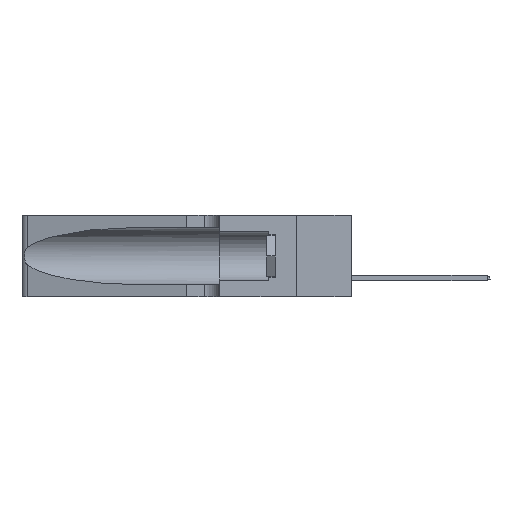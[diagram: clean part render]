
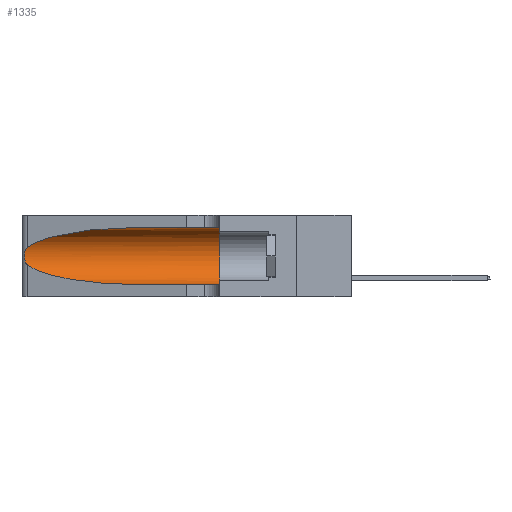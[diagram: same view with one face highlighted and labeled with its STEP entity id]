
A CAD part, left-side view. The second image highlights one B-rep face of the part: STEP entity #1335.
In plain terms, the highlighted cylindrical face has radius 3.308 mm (diameter 6.617 mm), a partial arc.
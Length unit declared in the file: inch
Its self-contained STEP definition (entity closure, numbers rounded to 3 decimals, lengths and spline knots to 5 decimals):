
#7 = CARTESIAN_POINT ( 'NONE',  ( 0.25487, 1.22718, 0.22369 ) ) ;
#128 = LINE ( 'NONE', #35612, #27657 ) ;
#715 = CARTESIAN_POINT ( 'NONE',  ( 0.25487, 1.22718, 0.14631 ) ) ;
#1195 = VERTEX_POINT ( 'NONE', #10495 ) ;
#1307 = VECTOR ( 'NONE', #25436, 39.37008 ) ;
#1335 = ADVANCED_FACE ( 'NONE', ( #28343 ), #4131, .F. ) ;
#1412 = EDGE_CURVE ( 'NONE', #36514, #11621, #7778, .T. ) ;
#1617 = CARTESIAN_POINT ( 'NONE',  ( 0.25487, 1.22718, 0.22369 ) ) ;
#1991 = CARTESIAN_POINT ( 'NONE',  ( 0.1305, 1.61858, 0.185 ) ) ;
#2319 = VERTEX_POINT ( 'NONE', #9872 ) ;
#2903 = CARTESIAN_POINT ( 'NONE',  ( 0.26075, 1.23896, 0.178 ) ) ;
#3033 = CARTESIAN_POINT ( 'NONE',  ( 0.25789, 1.23486, 0.15765 ) ) ;
#3961 = ORIENTED_EDGE ( 'NONE', *, *, #21579, .T. ) ;
#4131 = CYLINDRICAL_SURFACE ( 'NONE', #6169, 0.13025 ) ;
#5110 = EDGE_CURVE ( 'NONE', #11621, #1195, #24837, .T. ) ;
#5820 = CARTESIAN_POINT ( 'NONE',  ( 0.25856, 1.23593, 0.16098 ) ) ;
#6169 = AXIS2_PLACEMENT_3D ( 'NONE', #1991, #29302, #35127 ) ;
#6787 = EDGE_CURVE ( 'NONE', #37395, #30925, #23194, .T. ) ;
#6931 = ORIENTED_EDGE ( 'NONE', *, *, #1412, .T. ) ;
#7778 = B_SPLINE_CURVE_WITH_KNOTS ( 'NONE', 3,
 ( #29827, #20867, #11815, #27063, #18210, #35803, #11692, #2903, #17685, #5820, #3033, #33004, #18070, #21132 ),
 .UNSPECIFIED., .F., .F.,
 ( 4, 2, 2, 2, 2, 2, 4 ),
 ( 0., 0.00027, 0.00053, 0.00107, 0.0016, 0.00187, 0.00214 ),
 .UNSPECIFIED. ) ;
#8975 = CARTESIAN_POINT ( 'NONE',  ( 0.25487, 1.22718, 0.14631 ) ) ;
#9872 = CARTESIAN_POINT ( 'NONE',  ( 0.1305, 0.72297, 0.31525 ) ) ;
#10495 = CARTESIAN_POINT ( 'NONE',  ( 0.1305, 0.72297, 0.05475 ) ) ;
#11621 = VERTEX_POINT ( 'NONE', #715 ) ;
#11692 = CARTESIAN_POINT ( 'NONE',  ( 0.26075, 1.23896, 0.19203 ) ) ;
#11815 = CARTESIAN_POINT ( 'NONE',  ( 0.25639, 1.23184, 0.21858 ) ) ;
#16111 = EDGE_LOOP ( 'NONE', ( #3961, #6931, #22459, #38555, #16533, #20834 ) ) ;
#16533 = ORIENTED_EDGE ( 'NONE', *, *, #6787, .F. ) ;
#16592 = DIRECTION ( 'NONE',  ( 0., 0., 1. ) ) ;
#17495 = DIRECTION ( 'NONE',  ( 0., -1., 0. ) ) ;
#17685 = CARTESIAN_POINT ( 'NONE',  ( 0.26017, 1.23833, 0.17102 ) ) ;
#18070 = CARTESIAN_POINT ( 'NONE',  ( 0.25555, 1.22993, 0.14849 ) ) ;
#18191 = CARTESIAN_POINT ( 'NONE',  ( 0.1305, 0.35, 0.31525 ) ) ;
#18210 = CARTESIAN_POINT ( 'NONE',  ( 0.25854, 1.2359, 0.20912 ) ) ;
#18369 = CARTESIAN_POINT ( 'NONE',  ( 0.1305, 0.72297, 0.31525 ) ) ;
#20703 = CARTESIAN_POINT ( 'NONE',  ( 0.18966, 0.96281, 0.05475 ) ) ;
#20834 = ORIENTED_EDGE ( 'NONE', *, *, #35710, .F. ) ;
#20867 = CARTESIAN_POINT ( 'NONE',  ( 0.25555, 1.22994, 0.2215 ) ) ;
#21132 = CARTESIAN_POINT ( 'NONE',  ( 0.25487, 1.22718, 0.14631 ) ) ;
#21579 = EDGE_CURVE ( 'NONE', #2319, #36514, #34247, .T. ) ;
#22459 = ORIENTED_EDGE ( 'NONE', *, *, #5110, .T. ) ;
#23194 = CIRCLE ( 'NONE', #23865, 0.13025 ) ;
#23857 = CARTESIAN_POINT ( 'NONE',  ( 0.1305, 0.72297, 0.05475 ) ) ;
#23865 = AXIS2_PLACEMENT_3D ( 'NONE', #34685, #31256, #16592 ) ;
#24700 = CARTESIAN_POINT ( 'NONE',  ( 0.18966, 0.96281, 0.31525 ) ) ;
#24837 =( BOUNDED_CURVE ( )  B_SPLINE_CURVE ( 3, ( #8975, #36161, #20703, #23857 ),
 .UNSPECIFIED., .F., .F. ) 
 B_SPLINE_CURVE_WITH_KNOTS ( ( 4, 4 ),
 ( 3.44316, 4.71239 ),
 .UNSPECIFIED. ) 
 CURVE ( )  GEOMETRIC_REPRESENTATION_ITEM ( )  RATIONAL_B_SPLINE_CURVE ( ( 1., 0.87, 0.87, 1. ) ) 
 REPRESENTATION_ITEM ( '' )  );
#25436 = DIRECTION ( 'NONE',  ( 0., -1., 0. ) ) ;
#27063 = CARTESIAN_POINT ( 'NONE',  ( 0.25787, 1.23484, 0.2124 ) ) ;
#27657 = VECTOR ( 'NONE', #17495, 39.37008 ) ;
#27735 = CARTESIAN_POINT ( 'NONE',  ( 0.2373, 1.15595, 0.28018 ) ) ;
#28343 = FACE_OUTER_BOUND ( 'NONE', #16111, .T. ) ;
#28719 = CARTESIAN_POINT ( 'NONE',  ( 0.1305, 1.61858, 0.31525 ) ) ;
#29302 = DIRECTION ( 'NONE',  ( 0., -1., 0. ) ) ;
#29827 = CARTESIAN_POINT ( 'NONE',  ( 0.25487, 1.22718, 0.22369 ) ) ;
#30272 = EDGE_CURVE ( 'NONE', #1195, #30925, #128, .T. ) ;
#30730 = LINE ( 'NONE', #28719, #1307 ) ;
#30925 = VERTEX_POINT ( 'NONE', #33156 ) ;
#31256 = DIRECTION ( 'NONE',  ( 0., 1., 0. ) ) ;
#33004 = CARTESIAN_POINT ( 'NONE',  ( 0.25639, 1.23186, 0.15144 ) ) ;
#33156 = CARTESIAN_POINT ( 'NONE',  ( 0.1305, 0.35, 0.05475 ) ) ;
#34247 =( BOUNDED_CURVE ( )  B_SPLINE_CURVE ( 3, ( #18369, #24700, #27735, #7 ),
 .UNSPECIFIED., .F., .F. ) 
 B_SPLINE_CURVE_WITH_KNOTS ( ( 4, 4 ),
 ( 1.5708, 2.84003 ),
 .UNSPECIFIED. ) 
 CURVE ( )  GEOMETRIC_REPRESENTATION_ITEM ( )  RATIONAL_B_SPLINE_CURVE ( ( 1., 0.87, 0.87, 1. ) ) 
 REPRESENTATION_ITEM ( '' )  );
#34685 = CARTESIAN_POINT ( 'NONE',  ( 0.1305, 0.35, 0.185 ) ) ;
#35127 = DIRECTION ( 'NONE',  ( 0., 0., -1. ) ) ;
#35612 = CARTESIAN_POINT ( 'NONE',  ( 0.1305, 1.61858, 0.05475 ) ) ;
#35710 = EDGE_CURVE ( 'NONE', #2319, #37395, #30730, .T. ) ;
#35803 = CARTESIAN_POINT ( 'NONE',  ( 0.26018, 1.23835, 0.19895 ) ) ;
#36161 = CARTESIAN_POINT ( 'NONE',  ( 0.2373, 1.15595, 0.08982 ) ) ;
#36514 = VERTEX_POINT ( 'NONE', #1617 ) ;
#37395 = VERTEX_POINT ( 'NONE', #18191 ) ;
#38555 = ORIENTED_EDGE ( 'NONE', *, *, #30272, .T. ) ;
